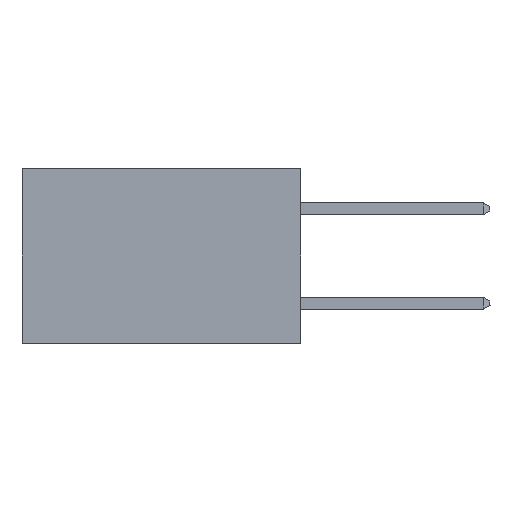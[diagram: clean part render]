
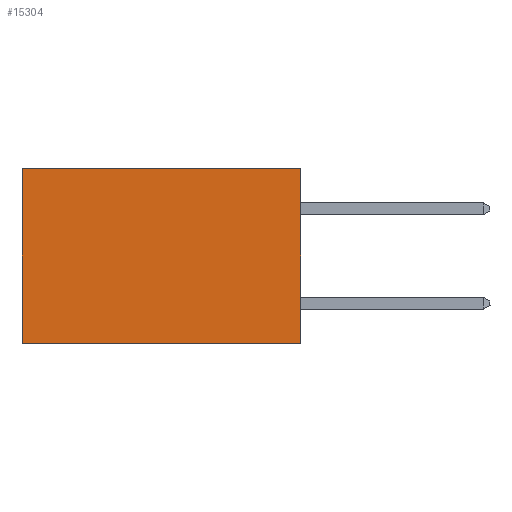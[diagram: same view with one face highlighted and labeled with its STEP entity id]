
A CAD part, left-side view. The second image highlights one B-rep face of the part: STEP entity #15304.
In plain terms, the highlighted planar face has unit normal (-1, 0, 0).
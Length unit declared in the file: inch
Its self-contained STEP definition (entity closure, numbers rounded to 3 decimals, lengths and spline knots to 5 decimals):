
#707 = DIRECTION ( 'NONE',  ( 0., 1., 0. ) ) ;
#777 = ORIENTED_EDGE ( 'NONE', *, *, #17373, .F. ) ;
#896 = ORIENTED_EDGE ( 'NONE', *, *, #11524, .T. ) ;
#1506 = DIRECTION ( 'NONE',  ( 0., 0., -1. ) ) ;
#2398 = DIRECTION ( 'NONE',  ( 0., 1., 0. ) ) ;
#3546 = CARTESIAN_POINT ( 'NONE',  ( 0.277, 0., 0. ) ) ;
#3861 = CARTESIAN_POINT ( 'NONE',  ( 0.277, 0.59, 0. ) ) ;
#4233 = VERTEX_POINT ( 'NONE', #16546 ) ;
#4341 = CARTESIAN_POINT ( 'NONE',  ( 0.277, 0.59, -0.37 ) ) ;
#5196 = ORIENTED_EDGE ( 'NONE', *, *, #6604, .T. ) ;
#5663 = FACE_OUTER_BOUND ( 'NONE', #13695, .T. ) ;
#6604 = EDGE_CURVE ( 'NONE', #15499, #16977, #12825, .T. ) ;
#7916 = EDGE_CURVE ( 'NONE', #9860, #4233, #13932, .T. ) ;
#8405 = CARTESIAN_POINT ( 'NONE',  ( 0.277, 0., -0.37 ) ) ;
#9860 = VERTEX_POINT ( 'NONE', #12852 ) ;
#10682 = AXIS2_PLACEMENT_3D ( 'NONE', #16531, #10683, #1506 ) ;
#10683 = DIRECTION ( 'NONE',  ( 1., 0., 0. ) ) ;
#10971 = ORIENTED_EDGE ( 'NONE', *, *, #7916, .F. ) ;
#11264 = VECTOR ( 'NONE', #15219, 39.37008 ) ;
#11524 = EDGE_CURVE ( 'NONE', #16977, #4233, #17658, .T. ) ;
#12127 = PLANE ( 'NONE',  #10682 ) ;
#12355 = VECTOR ( 'NONE', #2398, 39.37008 ) ;
#12825 = LINE ( 'NONE', #18804, #12355 ) ;
#12852 = CARTESIAN_POINT ( 'NONE',  ( 0.277, 0., -0.37 ) ) ;
#13695 = EDGE_LOOP ( 'NONE', ( #896, #10971, #777, #5196 ) ) ;
#13767 = CARTESIAN_POINT ( 'NONE',  ( 0.277, 0., -0.37 ) ) ;
#13932 = LINE ( 'NONE', #8405, #17773 ) ;
#15219 = DIRECTION ( 'NONE',  ( 0., 0., -1. ) ) ;
#15304 = ADVANCED_FACE ( 'NONE', ( #5663 ), #12127, .F. ) ;
#15499 = VERTEX_POINT ( 'NONE', #3546 ) ;
#16304 = DIRECTION ( 'NONE',  ( 0., 0., -1. ) ) ;
#16531 = CARTESIAN_POINT ( 'NONE',  ( 0.277, 0., -0.37 ) ) ;
#16546 = CARTESIAN_POINT ( 'NONE',  ( 0.277, 0.59, -0.37 ) ) ;
#16763 = VECTOR ( 'NONE', #16304, 39.37008 ) ;
#16977 = VERTEX_POINT ( 'NONE', #3861 ) ;
#17373 = EDGE_CURVE ( 'NONE', #15499, #9860, #19024, .T. ) ;
#17658 = LINE ( 'NONE', #4341, #16763 ) ;
#17773 = VECTOR ( 'NONE', #707, 39.37008 ) ;
#18804 = CARTESIAN_POINT ( 'NONE',  ( 0.277, 0., 0. ) ) ;
#19024 = LINE ( 'NONE', #13767, #11264 ) ;
